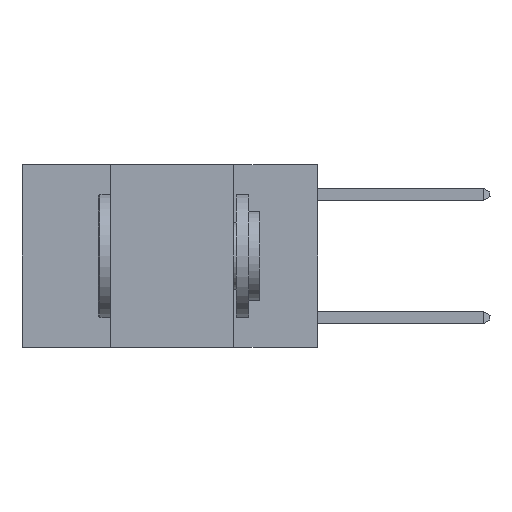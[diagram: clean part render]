
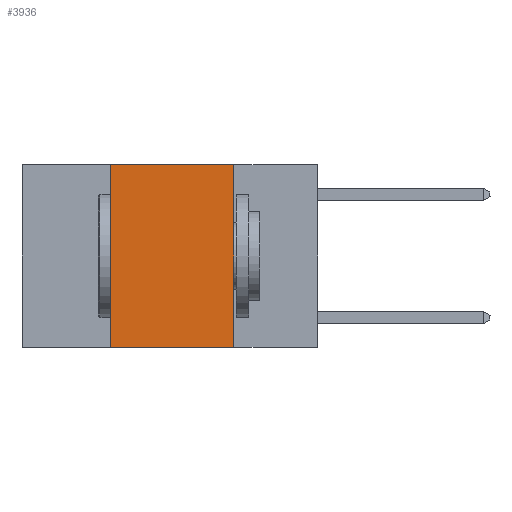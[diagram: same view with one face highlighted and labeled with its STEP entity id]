
A CAD part, left-side view. The second image highlights one B-rep face of the part: STEP entity #3936.
In plain terms, the highlighted planar face has unit normal (-1, 0, 0).
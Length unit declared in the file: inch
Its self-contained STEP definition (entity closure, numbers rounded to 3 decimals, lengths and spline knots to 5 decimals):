
#553 = DIRECTION ( 'NONE',  ( 1., 0., 0. ) ) ;
#573 = AXIS2_PLACEMENT_3D ( 'NONE', #10219, #553, #13584 ) ;
#722 = ORIENTED_EDGE ( 'NONE', *, *, #12927, .F. ) ;
#1094 = CARTESIAN_POINT ( 'NONE',  ( 0., 0.42, -0.37 ) ) ;
#1671 = CARTESIAN_POINT ( 'NONE',  ( 0., 0.17, 0. ) ) ;
#1832 = EDGE_CURVE ( 'NONE', #8289, #2124, #5026, .T. ) ;
#2074 = EDGE_CURVE ( 'NONE', #5226, #8289, #7681, .T. ) ;
#2124 = VERTEX_POINT ( 'NONE', #10386 ) ;
#2405 = EDGE_LOOP ( 'NONE', ( #9008, #7875, #722, #13616 ) ) ;
#2811 = CARTESIAN_POINT ( 'NONE',  ( 0., 0.6, -0.37 ) ) ;
#2965 = DIRECTION ( 'NONE',  ( 0., -1., 0. ) ) ;
#3854 = LINE ( 'NONE', #4014, #10751 ) ;
#3927 = DIRECTION ( 'NONE',  ( 0., 0., 1. ) ) ;
#3936 = ADVANCED_FACE ( 'NONE', ( #11297 ), #14951, .F. ) ;
#4014 = CARTESIAN_POINT ( 'NONE',  ( 0., 0.42, 0. ) ) ;
#4868 = DIRECTION ( 'NONE',  ( 0., 0., -1. ) ) ;
#5026 = LINE ( 'NONE', #7139, #9956 ) ;
#5226 = VERTEX_POINT ( 'NONE', #13907 ) ;
#6956 = EDGE_CURVE ( 'NONE', #11653, #2124, #13644, .T. ) ;
#7139 = CARTESIAN_POINT ( 'NONE',  ( 0., 0.17, 0. ) ) ;
#7681 = LINE ( 'NONE', #9934, #9708 ) ;
#7875 = ORIENTED_EDGE ( 'NONE', *, *, #2074, .F. ) ;
#8289 = VERTEX_POINT ( 'NONE', #1671 ) ;
#9008 = ORIENTED_EDGE ( 'NONE', *, *, #1832, .F. ) ;
#9708 = VECTOR ( 'NONE', #14967, 39.37008 ) ;
#9934 = CARTESIAN_POINT ( 'NONE',  ( 0., 0.6, 0. ) ) ;
#9956 = VECTOR ( 'NONE', #4868, 39.37008 ) ;
#10219 = CARTESIAN_POINT ( 'NONE',  ( 0., 0.6, 0. ) ) ;
#10386 = CARTESIAN_POINT ( 'NONE',  ( 0., 0.17, -0.37 ) ) ;
#10751 = VECTOR ( 'NONE', #3927, 39.37008 ) ;
#11297 = FACE_OUTER_BOUND ( 'NONE', #2405, .T. ) ;
#11653 = VERTEX_POINT ( 'NONE', #1094 ) ;
#12927 = EDGE_CURVE ( 'NONE', #11653, #5226, #3854, .T. ) ;
#13584 = DIRECTION ( 'NONE',  ( 0., 0., -1. ) ) ;
#13616 = ORIENTED_EDGE ( 'NONE', *, *, #6956, .T. ) ;
#13644 = LINE ( 'NONE', #2811, #15213 ) ;
#13907 = CARTESIAN_POINT ( 'NONE',  ( 0., 0.42, 0. ) ) ;
#14951 = PLANE ( 'NONE',  #573 ) ;
#14967 = DIRECTION ( 'NONE',  ( 0., -1., 0. ) ) ;
#15213 = VECTOR ( 'NONE', #2965, 39.37008 ) ;
